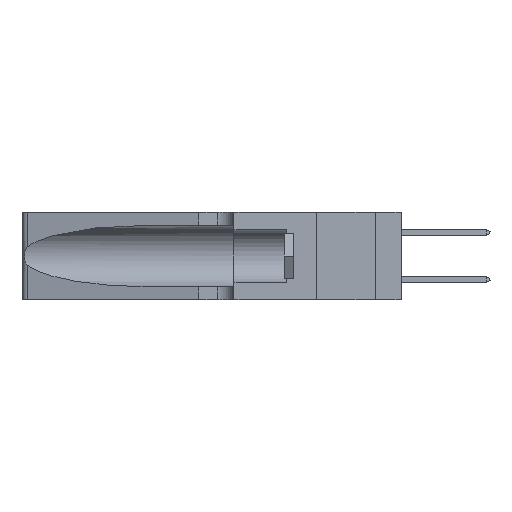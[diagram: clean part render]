
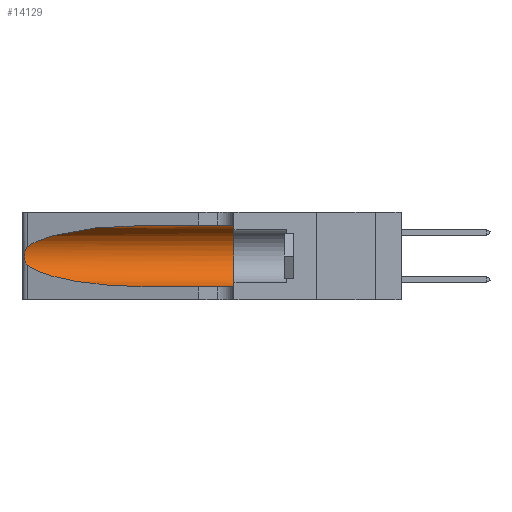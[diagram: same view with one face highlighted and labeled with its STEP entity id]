
A CAD part, left-side view. The second image highlights one B-rep face of the part: STEP entity #14129.
In plain terms, the highlighted cylindrical face has radius 3.308 mm (diameter 6.617 mm), a partial arc.
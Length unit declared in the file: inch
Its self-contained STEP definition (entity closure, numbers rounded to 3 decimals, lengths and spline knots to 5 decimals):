
#457 = CARTESIAN_POINT ( 'NONE',  ( 0.25856, 1.23593, 0.16098 ) ) ;
#764 = CARTESIAN_POINT ( 'NONE',  ( 0.25639, 1.23184, 0.21858 ) ) ;
#966 =( BOUNDED_CURVE ( )  B_SPLINE_CURVE ( 3, ( #15721, #11428, #20289, #10286 ),
 .UNSPECIFIED., .F., .F. ) 
 B_SPLINE_CURVE_WITH_KNOTS ( ( 4, 4 ),
 ( 1.5708, 2.84003 ),
 .UNSPECIFIED. ) 
 CURVE ( )  GEOMETRIC_REPRESENTATION_ITEM ( )  RATIONAL_B_SPLINE_CURVE ( ( 1., 0.87, 0.87, 1. ) ) 
 REPRESENTATION_ITEM ( '' )  );
#1438 = ORIENTED_EDGE ( 'NONE', *, *, #11054, .T. ) ;
#1520 = LINE ( 'NONE', #10676, #28763 ) ;
#2720 = CYLINDRICAL_SURFACE ( 'NONE', #2990, 0.13025 ) ;
#2909 = CARTESIAN_POINT ( 'NONE',  ( 0.26017, 1.23833, 0.17102 ) ) ;
#2990 = AXIS2_PLACEMENT_3D ( 'NONE', #18111, #27982, #5029 ) ;
#3016 = CARTESIAN_POINT ( 'NONE',  ( 0.25555, 1.22993, 0.14849 ) ) ;
#3224 = CARTESIAN_POINT ( 'NONE',  ( 0.26018, 1.23835, 0.19895 ) ) ;
#4833 = EDGE_CURVE ( 'NONE', #12250, #29206, #1520, .T. ) ;
#5029 = DIRECTION ( 'NONE',  ( 0., 0., -1. ) ) ;
#5163 = CARTESIAN_POINT ( 'NONE',  ( 0.25487, 1.22718, 0.22369 ) ) ;
#5273 = CARTESIAN_POINT ( 'NONE',  ( 0.25487, 1.22718, 0.14631 ) ) ;
#5431 = ORIENTED_EDGE ( 'NONE', *, *, #12706, .T. ) ;
#6081 = LINE ( 'NONE', #12149, #28263 ) ;
#6340 = VERTEX_POINT ( 'NONE', #15014 ) ;
#7258 = CARTESIAN_POINT ( 'NONE',  ( 0.1305, 0.35, 0.31525 ) ) ;
#10029 = ORIENTED_EDGE ( 'NONE', *, *, #4833, .F. ) ;
#10087 = B_SPLINE_CURVE_WITH_KNOTS ( 'NONE', 3,
 ( #5163, #17120, #764, #21476, #26384, #3224, #24015, #25967, #2909, #457, #12085, #19353, #3016, #21378 ),
 .UNSPECIFIED., .F., .F.,
 ( 4, 2, 2, 2, 2, 2, 4 ),
 ( 0., 0.00027, 0.00053, 0.00107, 0.0016, 0.00187, 0.00214 ),
 .UNSPECIFIED. ) ;
#10286 = CARTESIAN_POINT ( 'NONE',  ( 0.25487, 1.22718, 0.22369 ) ) ;
#10420 = ORIENTED_EDGE ( 'NONE', *, *, #20913, .T. ) ;
#10676 = CARTESIAN_POINT ( 'NONE',  ( 0.1305, 1.61858, 0.31525 ) ) ;
#10770 = CARTESIAN_POINT ( 'NONE',  ( 0.25487, 1.22718, 0.14631 ) ) ;
#11054 = EDGE_CURVE ( 'NONE', #12250, #6340, #966, .T. ) ;
#11428 = CARTESIAN_POINT ( 'NONE',  ( 0.18966, 0.96281, 0.31525 ) ) ;
#11953 = DIRECTION ( 'NONE',  ( 0., -1., 0. ) ) ;
#12085 = CARTESIAN_POINT ( 'NONE',  ( 0.25789, 1.23486, 0.15765 ) ) ;
#12128 = CARTESIAN_POINT ( 'NONE',  ( 0.1305, 0.35, 0.185 ) ) ;
#12149 = CARTESIAN_POINT ( 'NONE',  ( 0.1305, 1.61858, 0.05475 ) ) ;
#12250 = VERTEX_POINT ( 'NONE', #26012 ) ;
#12498 = CIRCLE ( 'NONE', #29148, 0.13025 ) ;
#12706 = EDGE_CURVE ( 'NONE', #23513, #18226, #6081, .T. ) ;
#13733 = VERTEX_POINT ( 'NONE', #10770 ) ;
#14129 = ADVANCED_FACE ( 'NONE', ( #28530 ), #2720, .F. ) ;
#14551 =( BOUNDED_CURVE ( )  B_SPLINE_CURVE ( 3, ( #5273, #14792, #19159, #19256 ),
 .UNSPECIFIED., .F., .F. ) 
 B_SPLINE_CURVE_WITH_KNOTS ( ( 4, 4 ),
 ( 3.44316, 4.71239 ),
 .UNSPECIFIED. ) 
 CURVE ( )  GEOMETRIC_REPRESENTATION_ITEM ( )  RATIONAL_B_SPLINE_CURVE ( ( 1., 0.87, 0.87, 1. ) ) 
 REPRESENTATION_ITEM ( '' )  );
#14736 = DIRECTION ( 'NONE',  ( 0., 1., 0. ) ) ;
#14792 = CARTESIAN_POINT ( 'NONE',  ( 0.2373, 1.15595, 0.08982 ) ) ;
#15014 = CARTESIAN_POINT ( 'NONE',  ( 0.25487, 1.22718, 0.22369 ) ) ;
#15355 = EDGE_CURVE ( 'NONE', #29206, #18226, #12498, .T. ) ;
#15721 = CARTESIAN_POINT ( 'NONE',  ( 0.1305, 0.72297, 0.31525 ) ) ;
#17120 = CARTESIAN_POINT ( 'NONE',  ( 0.25555, 1.22994, 0.2215 ) ) ;
#18111 = CARTESIAN_POINT ( 'NONE',  ( 0.1305, 1.61858, 0.185 ) ) ;
#18226 = VERTEX_POINT ( 'NONE', #25139 ) ;
#19159 = CARTESIAN_POINT ( 'NONE',  ( 0.18966, 0.96281, 0.05475 ) ) ;
#19256 = CARTESIAN_POINT ( 'NONE',  ( 0.1305, 0.72297, 0.05475 ) ) ;
#19353 = CARTESIAN_POINT ( 'NONE',  ( 0.25639, 1.23186, 0.15144 ) ) ;
#19656 = ORIENTED_EDGE ( 'NONE', *, *, #20910, .T. ) ;
#20289 = CARTESIAN_POINT ( 'NONE',  ( 0.2373, 1.15595, 0.28018 ) ) ;
#20910 = EDGE_CURVE ( 'NONE', #6340, #13733, #10087, .T. ) ;
#20913 = EDGE_CURVE ( 'NONE', #13733, #23513, #14551, .T. ) ;
#21378 = CARTESIAN_POINT ( 'NONE',  ( 0.25487, 1.22718, 0.14631 ) ) ;
#21476 = CARTESIAN_POINT ( 'NONE',  ( 0.25787, 1.23484, 0.2124 ) ) ;
#22690 = ORIENTED_EDGE ( 'NONE', *, *, #15355, .F. ) ;
#22855 = CARTESIAN_POINT ( 'NONE',  ( 0.1305, 0.72297, 0.05475 ) ) ;
#23513 = VERTEX_POINT ( 'NONE', #22855 ) ;
#24015 = CARTESIAN_POINT ( 'NONE',  ( 0.26075, 1.23896, 0.19203 ) ) ;
#25077 = EDGE_LOOP ( 'NONE', ( #1438, #19656, #10420, #5431, #22690, #10029 ) ) ;
#25139 = CARTESIAN_POINT ( 'NONE',  ( 0.1305, 0.35, 0.05475 ) ) ;
#25967 = CARTESIAN_POINT ( 'NONE',  ( 0.26075, 1.23896, 0.178 ) ) ;
#26012 = CARTESIAN_POINT ( 'NONE',  ( 0.1305, 0.72297, 0.31525 ) ) ;
#26189 = DIRECTION ( 'NONE',  ( 0., -1., 0. ) ) ;
#26219 = DIRECTION ( 'NONE',  ( 0., 0., 1. ) ) ;
#26384 = CARTESIAN_POINT ( 'NONE',  ( 0.25854, 1.2359, 0.20912 ) ) ;
#27982 = DIRECTION ( 'NONE',  ( 0., -1., 0. ) ) ;
#28263 = VECTOR ( 'NONE', #11953, 39.37008 ) ;
#28530 = FACE_OUTER_BOUND ( 'NONE', #25077, .T. ) ;
#28763 = VECTOR ( 'NONE', #26189, 39.37008 ) ;
#29148 = AXIS2_PLACEMENT_3D ( 'NONE', #12128, #14736, #26219 ) ;
#29206 = VERTEX_POINT ( 'NONE', #7258 ) ;
